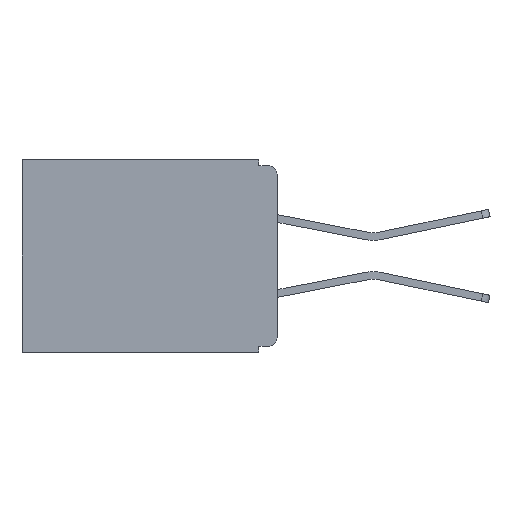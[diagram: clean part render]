
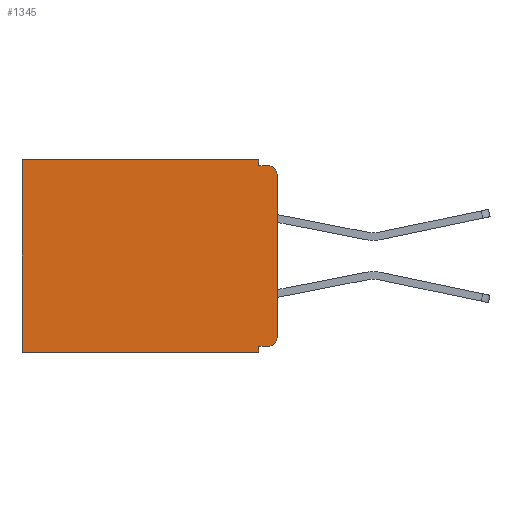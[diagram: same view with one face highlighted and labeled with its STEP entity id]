
A CAD part, left-side view. The second image highlights one B-rep face of the part: STEP entity #1345.
In plain terms, the highlighted planar face has unit normal (-1, 0, 0).
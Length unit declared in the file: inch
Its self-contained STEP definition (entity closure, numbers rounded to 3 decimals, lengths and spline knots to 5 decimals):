
#715 = CIRCLE ( 'NONE', #21967, 0.015 ) ;
#1109 = LINE ( 'NONE', #8038, #19883 ) ;
#1345 = ADVANCED_FACE ( 'NONE', ( #27596 ), #11185, .F. ) ;
#2084 = DIRECTION ( 'NONE',  ( 0., 0., -1. ) ) ;
#2149 = AXIS2_PLACEMENT_3D ( 'NONE', #6238, #23037, #8738 ) ;
#3179 = CARTESIAN_POINT ( 'NONE',  ( 0.3, 0., -0.33 ) ) ;
#4275 = DIRECTION ( 'NONE',  ( 0., -1., 0. ) ) ;
#5068 = EDGE_CURVE ( 'NONE', #18945, #8510, #10679, .T. ) ;
#5524 = EDGE_CURVE ( 'NONE', #8510, #27954, #17735, .T. ) ;
#5817 = CARTESIAN_POINT ( 'NONE',  ( 0.3, 0.437, -0.33 ) ) ;
#6081 = DIRECTION ( 'NONE',  ( 0., 0., -1. ) ) ;
#6238 = CARTESIAN_POINT ( 'NONE',  ( 0.3, 0.015, -0.305 ) ) ;
#6981 = CARTESIAN_POINT ( 'NONE',  ( 0.3, 0., -0.305 ) ) ;
#7005 = CARTESIAN_POINT ( 'NONE',  ( 0.3, 0.015, -0.025 ) ) ;
#8038 = CARTESIAN_POINT ( 'NONE',  ( 0.3, 0., -0.32 ) ) ;
#8124 = ORIENTED_EDGE ( 'NONE', *, *, #28042, .T. ) ;
#8239 = ORIENTED_EDGE ( 'NONE', *, *, #5068, .F. ) ;
#8510 = VERTEX_POINT ( 'NONE', #14909 ) ;
#8617 = CARTESIAN_POINT ( 'NONE',  ( 0.3, 0.031, -0.33 ) ) ;
#8738 = DIRECTION ( 'NONE',  ( 0., 0., -1. ) ) ;
#8945 = CARTESIAN_POINT ( 'NONE',  ( 0.3, 0.031, 0. ) ) ;
#9262 = EDGE_CURVE ( 'NONE', #10410, #16838, #22263, .T. ) ;
#9512 = DIRECTION ( 'NONE',  ( 0., 0., -1. ) ) ;
#9659 = DIRECTION ( 'NONE',  ( 0., 0., -1. ) ) ;
#9984 = EDGE_CURVE ( 'NONE', #22317, #14668, #715, .T. ) ;
#10410 = VERTEX_POINT ( 'NONE', #21044 ) ;
#10679 = LINE ( 'NONE', #8617, #22532 ) ;
#11185 = PLANE ( 'NONE',  #26966 ) ;
#11206 = CIRCLE ( 'NONE', #2149, 0.015 ) ;
#11216 = EDGE_CURVE ( 'NONE', #16838, #27954, #16151, .T. ) ;
#11390 = VECTOR ( 'NONE', #24983, 39.37008 ) ;
#12666 = ORIENTED_EDGE ( 'NONE', *, *, #24721, .F. ) ;
#13312 = CARTESIAN_POINT ( 'NONE',  ( 0.3, 0., -0.025 ) ) ;
#13359 = EDGE_CURVE ( 'NONE', #10410, #21337, #30386, .T. ) ;
#13422 = ORIENTED_EDGE ( 'NONE', *, *, #26895, .F. ) ;
#14438 = CARTESIAN_POINT ( 'NONE',  ( 0.3, 0.437, -0.33 ) ) ;
#14541 = CARTESIAN_POINT ( 'NONE',  ( 0.3, 0.015, -0.32 ) ) ;
#14668 = VERTEX_POINT ( 'NONE', #19025 ) ;
#14909 = CARTESIAN_POINT ( 'NONE',  ( 0.3, 0.031, -0.33 ) ) ;
#15436 = VECTOR ( 'NONE', #9659, 39.37008 ) ;
#15567 = DIRECTION ( 'NONE',  ( 0., 1., 0. ) ) ;
#15600 = CARTESIAN_POINT ( 'NONE',  ( 0.3, 0., 0. ) ) ;
#16151 = LINE ( 'NONE', #14438, #15436 ) ;
#16553 = ORIENTED_EDGE ( 'NONE', *, *, #5524, .F. ) ;
#16838 = VERTEX_POINT ( 'NONE', #30201 ) ;
#16927 = LINE ( 'NONE', #30602, #22401 ) ;
#17735 = LINE ( 'NONE', #25111, #11390 ) ;
#17790 = LINE ( 'NONE', #3179, #30309 ) ;
#18272 = VERTEX_POINT ( 'NONE', #6981 ) ;
#18710 = ORIENTED_EDGE ( 'NONE', *, *, #11216, .T. ) ;
#18945 = VERTEX_POINT ( 'NONE', #23119 ) ;
#19025 = CARTESIAN_POINT ( 'NONE',  ( 0.3, 0.015, -0.01 ) ) ;
#19687 = ORIENTED_EDGE ( 'NONE', *, *, #13359, .F. ) ;
#19820 = VERTEX_POINT ( 'NONE', #14541 ) ;
#19883 = VECTOR ( 'NONE', #24725, 39.37008 ) ;
#20215 = DIRECTION ( 'NONE',  ( 0., 0., -1. ) ) ;
#20802 = ORIENTED_EDGE ( 'NONE', *, *, #25872, .F. ) ;
#21044 = CARTESIAN_POINT ( 'NONE',  ( 0.3, 0.031, 0. ) ) ;
#21337 = VERTEX_POINT ( 'NONE', #28737 ) ;
#21534 = VECTOR ( 'NONE', #15567, 39.37008 ) ;
#21967 = AXIS2_PLACEMENT_3D ( 'NONE', #7005, #23762, #9512 ) ;
#22263 = LINE ( 'NONE', #15600, #21534 ) ;
#22317 = VERTEX_POINT ( 'NONE', #13312 ) ;
#22401 = VECTOR ( 'NONE', #4275, 39.37008 ) ;
#22532 = VECTOR ( 'NONE', #6081, 39.37008 ) ;
#23037 = DIRECTION ( 'NONE',  ( -1., 0., 0. ) ) ;
#23119 = CARTESIAN_POINT ( 'NONE',  ( 0.3, 0.031, -0.32 ) ) ;
#23226 = DIRECTION ( 'NONE',  ( 0., 0., -1. ) ) ;
#23762 = DIRECTION ( 'NONE',  ( -1., 0., 0. ) ) ;
#24078 = EDGE_LOOP ( 'NONE', ( #12666, #28924, #13422, #19687, #25618, #18710, #16553, #8239, #20802, #8124 ) ) ;
#24721 = EDGE_CURVE ( 'NONE', #22317, #18272, #17790, .T. ) ;
#24725 = DIRECTION ( 'NONE',  ( 0., 1., 0. ) ) ;
#24983 = DIRECTION ( 'NONE',  ( 0., 1., 0. ) ) ;
#25111 = CARTESIAN_POINT ( 'NONE',  ( 0.3, 0., -0.33 ) ) ;
#25618 = ORIENTED_EDGE ( 'NONE', *, *, #9262, .T. ) ;
#25872 = EDGE_CURVE ( 'NONE', #19820, #18945, #1109, .T. ) ;
#26895 = EDGE_CURVE ( 'NONE', #21337, #14668, #16927, .T. ) ;
#26966 = AXIS2_PLACEMENT_3D ( 'NONE', #28036, #30205, #2084 ) ;
#27596 = FACE_OUTER_BOUND ( 'NONE', #24078, .T. ) ;
#27954 = VERTEX_POINT ( 'NONE', #5817 ) ;
#28036 = CARTESIAN_POINT ( 'NONE',  ( 0.3, 0., -0.33 ) ) ;
#28042 = EDGE_CURVE ( 'NONE', #19820, #18272, #11206, .T. ) ;
#28737 = CARTESIAN_POINT ( 'NONE',  ( 0.3, 0.031, -0.01 ) ) ;
#28924 = ORIENTED_EDGE ( 'NONE', *, *, #9984, .T. ) ;
#29653 = VECTOR ( 'NONE', #23226, 39.37008 ) ;
#30201 = CARTESIAN_POINT ( 'NONE',  ( 0.3, 0.437, 0. ) ) ;
#30205 = DIRECTION ( 'NONE',  ( 1., 0., 0. ) ) ;
#30309 = VECTOR ( 'NONE', #20215, 39.37008 ) ;
#30386 = LINE ( 'NONE', #8945, #29653 ) ;
#30602 = CARTESIAN_POINT ( 'NONE',  ( 0.3, 0., -0.01 ) ) ;
